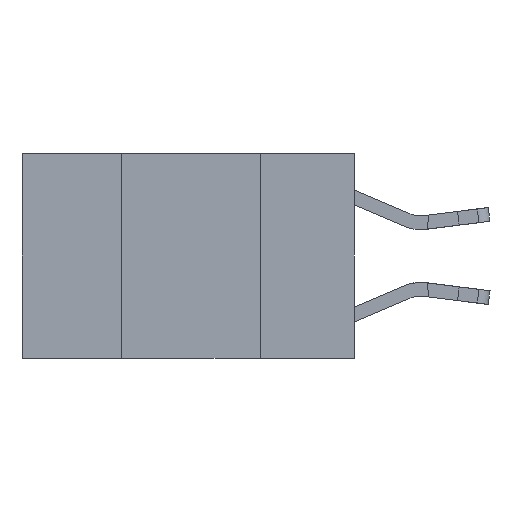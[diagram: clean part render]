
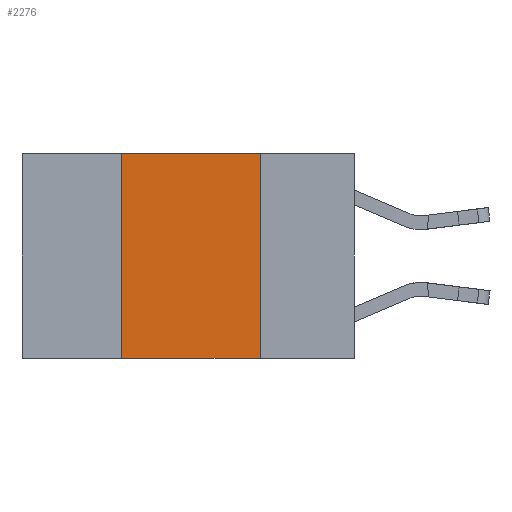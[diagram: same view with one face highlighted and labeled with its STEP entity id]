
A CAD part, left-side view. The second image highlights one B-rep face of the part: STEP entity #2276.
In plain terms, the highlighted planar face has unit normal (-1, 0, 0).
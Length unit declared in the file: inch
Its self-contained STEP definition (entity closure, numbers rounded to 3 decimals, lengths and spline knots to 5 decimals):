
#702 = CARTESIAN_POINT ( 'NONE',  ( 0., 0.42, 0. ) ) ;
#815 = LINE ( 'NONE', #6417, #4698 ) ;
#899 = ORIENTED_EDGE ( 'NONE', *, *, #17541, .F. ) ;
#1274 = FACE_OUTER_BOUND ( 'NONE', #22166, .T. ) ;
#1698 = CARTESIAN_POINT ( 'NONE',  ( 0., 0.6, 0. ) ) ;
#2276 = ADVANCED_FACE ( 'NONE', ( #1274 ), #13904, .F. ) ;
#3279 = DIRECTION ( 'NONE',  ( 0., 0., -1. ) ) ;
#3675 = DIRECTION ( 'NONE',  ( 0., -1., 0. ) ) ;
#4698 = VECTOR ( 'NONE', #8934, 39.37008 ) ;
#5564 = ORIENTED_EDGE ( 'NONE', *, *, #16235, .T. ) ;
#6417 = CARTESIAN_POINT ( 'NONE',  ( 0., 0.42, 0. ) ) ;
#7337 = VERTEX_POINT ( 'NONE', #20614 ) ;
#7809 = LINE ( 'NONE', #1698, #13986 ) ;
#8442 = VECTOR ( 'NONE', #19404, 39.37008 ) ;
#8934 = DIRECTION ( 'NONE',  ( 0., 0., 1. ) ) ;
#9921 = DIRECTION ( 'NONE',  ( 1., 0., 0. ) ) ;
#10130 = VERTEX_POINT ( 'NONE', #24947 ) ;
#10578 = VECTOR ( 'NONE', #3675, 39.37008 ) ;
#13503 = LINE ( 'NONE', #20997, #10578 ) ;
#13635 = CARTESIAN_POINT ( 'NONE',  ( 0., 0.6, 0. ) ) ;
#13904 = PLANE ( 'NONE',  #19198 ) ;
#13986 = VECTOR ( 'NONE', #16221, 39.37008 ) ;
#16221 = DIRECTION ( 'NONE',  ( 0., -1., 0. ) ) ;
#16235 = EDGE_CURVE ( 'NONE', #10130, #7337, #13503, .T. ) ;
#16996 = ORIENTED_EDGE ( 'NONE', *, *, #22966, .F. ) ;
#17541 = EDGE_CURVE ( 'NONE', #22062, #7337, #23104, .T. ) ;
#19184 = EDGE_CURVE ( 'NONE', #10130, #23854, #815, .T. ) ;
#19198 = AXIS2_PLACEMENT_3D ( 'NONE', #13635, #9921, #3279 ) ;
#19274 = CARTESIAN_POINT ( 'NONE',  ( 0., 0.17, 0. ) ) ;
#19404 = DIRECTION ( 'NONE',  ( 0., 0., -1. ) ) ;
#20614 = CARTESIAN_POINT ( 'NONE',  ( 0., 0.17, -0.37 ) ) ;
#20997 = CARTESIAN_POINT ( 'NONE',  ( 0., 0.6, -0.37 ) ) ;
#22062 = VERTEX_POINT ( 'NONE', #25835 ) ;
#22166 = EDGE_LOOP ( 'NONE', ( #899, #16996, #25978, #5564 ) ) ;
#22966 = EDGE_CURVE ( 'NONE', #23854, #22062, #7809, .T. ) ;
#23104 = LINE ( 'NONE', #19274, #8442 ) ;
#23854 = VERTEX_POINT ( 'NONE', #702 ) ;
#24947 = CARTESIAN_POINT ( 'NONE',  ( 0., 0.42, -0.37 ) ) ;
#25835 = CARTESIAN_POINT ( 'NONE',  ( 0., 0.17, 0. ) ) ;
#25978 = ORIENTED_EDGE ( 'NONE', *, *, #19184, .F. ) ;
